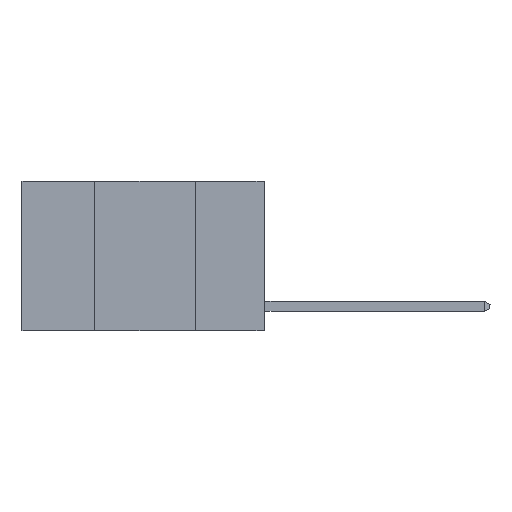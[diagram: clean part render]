
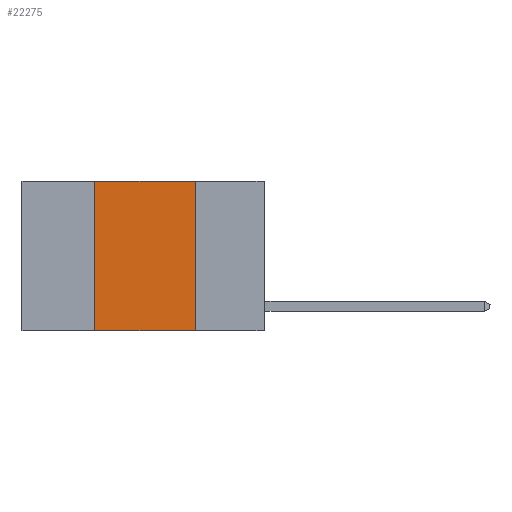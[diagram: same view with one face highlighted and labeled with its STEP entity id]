
A CAD part, left-side view. The second image highlights one B-rep face of the part: STEP entity #22275.
In plain terms, the highlighted planar face has unit normal (-1, 0, 0).
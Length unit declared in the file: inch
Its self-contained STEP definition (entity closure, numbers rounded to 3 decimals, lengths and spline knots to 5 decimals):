
#234 = CARTESIAN_POINT ( 'NONE',  ( 0., 0.6, 0. ) ) ;
#487 = CARTESIAN_POINT ( 'NONE',  ( 0., 0.6, -0.37 ) ) ;
#529 = EDGE_CURVE ( 'NONE', #15185, #17166, #16160, .T. ) ;
#2750 = DIRECTION ( 'NONE',  ( 0., 0., 1. ) ) ;
#2823 = EDGE_CURVE ( 'NONE', #20232, #13655, #24358, .T. ) ;
#3289 = DIRECTION ( 'NONE',  ( 0., -1., 0. ) ) ;
#4345 = DIRECTION ( 'NONE',  ( 0., 0., -1. ) ) ;
#4411 = ORIENTED_EDGE ( 'NONE', *, *, #529, .F. ) ;
#5123 = VECTOR ( 'NONE', #25192, 39.37008 ) ;
#6759 = LINE ( 'NONE', #20803, #11436 ) ;
#8474 = EDGE_CURVE ( 'NONE', #13655, #15185, #6759, .T. ) ;
#8897 = EDGE_CURVE ( 'NONE', #20232, #17166, #23369, .T. ) ;
#9062 = CARTESIAN_POINT ( 'NONE',  ( 0., 0.17, 0. ) ) ;
#10749 = CARTESIAN_POINT ( 'NONE',  ( 0., 0.42, 0. ) ) ;
#11086 = ORIENTED_EDGE ( 'NONE', *, *, #2823, .F. ) ;
#11436 = VECTOR ( 'NONE', #3289, 39.37008 ) ;
#12143 = ORIENTED_EDGE ( 'NONE', *, *, #8474, .F. ) ;
#13655 = VERTEX_POINT ( 'NONE', #21410 ) ;
#14087 = CARTESIAN_POINT ( 'NONE',  ( 0., 0.17, -0.37 ) ) ;
#14707 = AXIS2_PLACEMENT_3D ( 'NONE', #234, #16101, #4345 ) ;
#15185 = VERTEX_POINT ( 'NONE', #9062 ) ;
#15776 = CARTESIAN_POINT ( 'NONE',  ( 0., 0.42, -0.37 ) ) ;
#15918 = CARTESIAN_POINT ( 'NONE',  ( 0., 0.17, 0. ) ) ;
#16101 = DIRECTION ( 'NONE',  ( 1., 0., 0. ) ) ;
#16160 = LINE ( 'NONE', #15918, #5123 ) ;
#17166 = VERTEX_POINT ( 'NONE', #14087 ) ;
#18241 = DIRECTION ( 'NONE',  ( 0., -1., 0. ) ) ;
#18299 = VECTOR ( 'NONE', #18241, 39.37008 ) ;
#18356 = FACE_OUTER_BOUND ( 'NONE', #22819, .T. ) ;
#18723 = ORIENTED_EDGE ( 'NONE', *, *, #8897, .T. ) ;
#19316 = VECTOR ( 'NONE', #2750, 39.37008 ) ;
#19852 = PLANE ( 'NONE',  #14707 ) ;
#20232 = VERTEX_POINT ( 'NONE', #15776 ) ;
#20803 = CARTESIAN_POINT ( 'NONE',  ( 0., 0.6, 0. ) ) ;
#21410 = CARTESIAN_POINT ( 'NONE',  ( 0., 0.42, 0. ) ) ;
#22275 = ADVANCED_FACE ( 'NONE', ( #18356 ), #19852, .F. ) ;
#22819 = EDGE_LOOP ( 'NONE', ( #4411, #12143, #11086, #18723 ) ) ;
#23369 = LINE ( 'NONE', #487, #18299 ) ;
#24358 = LINE ( 'NONE', #10749, #19316 ) ;
#25192 = DIRECTION ( 'NONE',  ( 0., 0., -1. ) ) ;
